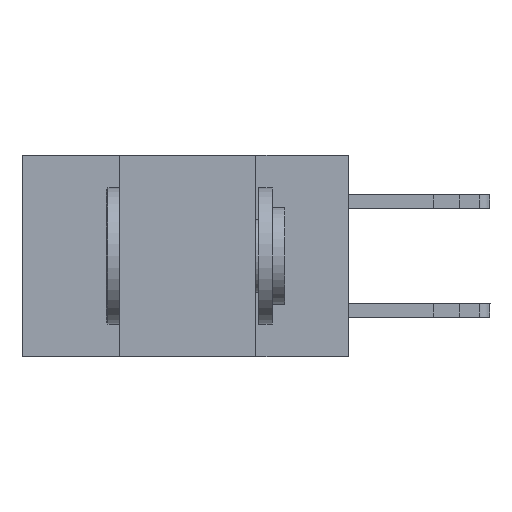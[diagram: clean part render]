
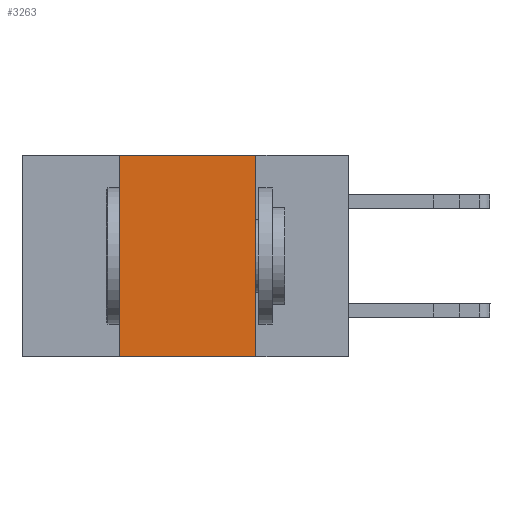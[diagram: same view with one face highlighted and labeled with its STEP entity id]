
A CAD part, left-side view. The second image highlights one B-rep face of the part: STEP entity #3263.
In plain terms, the highlighted planar face has unit normal (-1, 0, 0).
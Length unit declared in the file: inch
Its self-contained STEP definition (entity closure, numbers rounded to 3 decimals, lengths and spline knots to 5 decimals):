
#590 = FACE_OUTER_BOUND ( 'NONE', #16926, .T. ) ;
#657 = DIRECTION ( 'NONE',  ( 0., -1., 0. ) ) ;
#747 = VERTEX_POINT ( 'NONE', #6622 ) ;
#777 = CARTESIAN_POINT ( 'NONE',  ( 0., 0.6, -0.37 ) ) ;
#1802 = EDGE_CURVE ( 'NONE', #747, #6827, #17577, .T. ) ;
#3263 = ADVANCED_FACE ( 'NONE', ( #590 ), #14793, .F. ) ;
#4527 = VERTEX_POINT ( 'NONE', #16951 ) ;
#4579 = DIRECTION ( 'NONE',  ( 0., 0., 1. ) ) ;
#4688 = ORIENTED_EDGE ( 'NONE', *, *, #11028, .F. ) ;
#4847 = EDGE_CURVE ( 'NONE', #4527, #6827, #12947, .T. ) ;
#4873 = ORIENTED_EDGE ( 'NONE', *, *, #1802, .T. ) ;
#5485 = CARTESIAN_POINT ( 'NONE',  ( 0., 0.6, 0. ) ) ;
#5816 = AXIS2_PLACEMENT_3D ( 'NONE', #14751, #14696, #14671 ) ;
#6622 = CARTESIAN_POINT ( 'NONE',  ( 0., 0.42, -0.37 ) ) ;
#6827 = VERTEX_POINT ( 'NONE', #9237 ) ;
#6851 = VECTOR ( 'NONE', #4579, 39.37008 ) ;
#7880 = ORIENTED_EDGE ( 'NONE', *, *, #4847, .F. ) ;
#8310 = CARTESIAN_POINT ( 'NONE',  ( 0., 0.42, 0. ) ) ;
#8346 = VECTOR ( 'NONE', #12608, 39.37008 ) ;
#8484 = LINE ( 'NONE', #5485, #15475 ) ;
#8663 = CARTESIAN_POINT ( 'NONE',  ( 0., 0.42, -0.37 ) ) ;
#9168 = EDGE_CURVE ( 'NONE', #747, #13004, #17889, .T. ) ;
#9237 = CARTESIAN_POINT ( 'NONE',  ( 0., 0.17, -0.37 ) ) ;
#9599 = DIRECTION ( 'NONE',  ( 0., -1., 0. ) ) ;
#10738 = CARTESIAN_POINT ( 'NONE',  ( 0., 0.17, -0.37 ) ) ;
#11028 = EDGE_CURVE ( 'NONE', #13004, #4527, #8484, .T. ) ;
#11755 = ORIENTED_EDGE ( 'NONE', *, *, #9168, .F. ) ;
#12608 = DIRECTION ( 'NONE',  ( 0., 0., -1. ) ) ;
#12947 = LINE ( 'NONE', #10738, #8346 ) ;
#13004 = VERTEX_POINT ( 'NONE', #8310 ) ;
#13905 = VECTOR ( 'NONE', #657, 39.37008 ) ;
#14671 = DIRECTION ( 'NONE',  ( 0., 0., -1. ) ) ;
#14696 = DIRECTION ( 'NONE',  ( 1., 0., 0. ) ) ;
#14751 = CARTESIAN_POINT ( 'NONE',  ( 0., 0.6, 0. ) ) ;
#14793 = PLANE ( 'NONE',  #5816 ) ;
#15475 = VECTOR ( 'NONE', #9599, 39.37008 ) ;
#16926 = EDGE_LOOP ( 'NONE', ( #7880, #4688, #11755, #4873 ) ) ;
#16951 = CARTESIAN_POINT ( 'NONE',  ( 0., 0.17, 0. ) ) ;
#17577 = LINE ( 'NONE', #777, #13905 ) ;
#17889 = LINE ( 'NONE', #8663, #6851 ) ;
